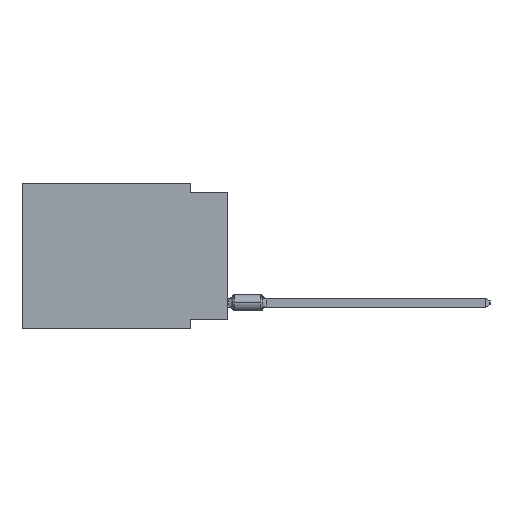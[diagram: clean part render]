
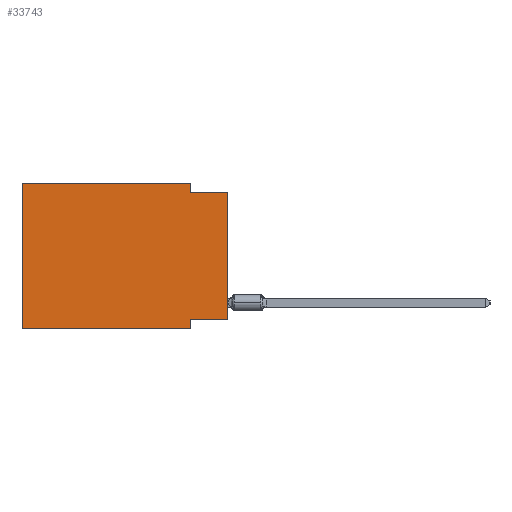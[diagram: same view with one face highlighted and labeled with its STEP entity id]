
A CAD part, left-side view. The second image highlights one B-rep face of the part: STEP entity #33743.
In plain terms, the highlighted planar face has unit normal (-1, 0, 0).
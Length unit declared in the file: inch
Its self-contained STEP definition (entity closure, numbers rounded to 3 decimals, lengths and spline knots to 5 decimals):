
#637 = CARTESIAN_POINT ( 'NONE',  ( 0., 0.55, 0. ) ) ;
#720 = DIRECTION ( 'NONE',  ( 0., 0., 1. ) ) ;
#764 = CARTESIAN_POINT ( 'NONE',  ( 0., 0.55, 0. ) ) ;
#1019 = CARTESIAN_POINT ( 'NONE',  ( 0., 0., -0.365 ) ) ;
#1382 = ORIENTED_EDGE ( 'NONE', *, *, #21105, .F. ) ;
#1525 = DIRECTION ( 'NONE',  ( 0., 0., -1. ) ) ;
#1823 = VERTEX_POINT ( 'NONE', #637 ) ;
#2099 = CARTESIAN_POINT ( 'NONE',  ( 0., 0.55, -0.39 ) ) ;
#2282 = CARTESIAN_POINT ( 'NONE',  ( 0., 0.55, 0. ) ) ;
#2800 = LINE ( 'NONE', #2282, #27940 ) ;
#3348 = LINE ( 'NONE', #8285, #8511 ) ;
#3445 = VECTOR ( 'NONE', #25038, 39.37008 ) ;
#4300 = ORIENTED_EDGE ( 'NONE', *, *, #12586, .T. ) ;
#5215 = VECTOR ( 'NONE', #23584, 39.37008 ) ;
#5415 = VERTEX_POINT ( 'NONE', #30188 ) ;
#5670 = VECTOR ( 'NONE', #11538, 39.37008 ) ;
#6249 = VECTOR ( 'NONE', #32378, 39.37008 ) ;
#6464 = EDGE_CURVE ( 'NONE', #22963, #1823, #2800, .T. ) ;
#7119 = VECTOR ( 'NONE', #720, 39.37008 ) ;
#8180 = ORIENTED_EDGE ( 'NONE', *, *, #17267, .F. ) ;
#8285 = CARTESIAN_POINT ( 'NONE',  ( 0., 0.1, -0.39 ) ) ;
#8511 = VECTOR ( 'NONE', #24791, 39.37008 ) ;
#9815 = CARTESIAN_POINT ( 'NONE',  ( 0., 0.1, 0. ) ) ;
#9948 = VERTEX_POINT ( 'NONE', #30672 ) ;
#10771 = VECTOR ( 'NONE', #1525, 39.37008 ) ;
#10955 = LINE ( 'NONE', #764, #6249 ) ;
#11538 = DIRECTION ( 'NONE',  ( 0., -1., 0. ) ) ;
#12586 = EDGE_CURVE ( 'NONE', #22963, #5415, #14336, .T. ) ;
#12925 = LINE ( 'NONE', #23476, #10771 ) ;
#13226 = LINE ( 'NONE', #26566, #5215 ) ;
#14336 = LINE ( 'NONE', #27322, #3445 ) ;
#15094 = ORIENTED_EDGE ( 'NONE', *, *, #21496, .F. ) ;
#15326 = EDGE_CURVE ( 'NONE', #25270, #18817, #27583, .T. ) ;
#15428 = PLANE ( 'NONE',  #31967 ) ;
#15624 = CARTESIAN_POINT ( 'NONE',  ( 0., 0.1, -0.365 ) ) ;
#15827 = EDGE_CURVE ( 'NONE', #24851, #9948, #12925, .T. ) ;
#15851 = EDGE_LOOP ( 'NONE', ( #25285, #20115, #17676, #1382, #32858, #4300, #15094, #8180 ) ) ;
#16592 = EDGE_CURVE ( 'NONE', #9948, #18817, #21894, .T. ) ;
#17267 = EDGE_CURVE ( 'NONE', #25270, #21760, #13226, .T. ) ;
#17676 = ORIENTED_EDGE ( 'NONE', *, *, #15827, .F. ) ;
#18791 = DIRECTION ( 'NONE',  ( 0., 0., 1. ) ) ;
#18817 = VERTEX_POINT ( 'NONE', #23208 ) ;
#20115 = ORIENTED_EDGE ( 'NONE', *, *, #16592, .F. ) ;
#21105 = EDGE_CURVE ( 'NONE', #1823, #24851, #10955, .T. ) ;
#21496 = EDGE_CURVE ( 'NONE', #21760, #5415, #3348, .T. ) ;
#21549 = CARTESIAN_POINT ( 'NONE',  ( 0., 0., -0.025 ) ) ;
#21760 = VERTEX_POINT ( 'NONE', #15624 ) ;
#21894 = LINE ( 'NONE', #21549, #5670 ) ;
#22963 = VERTEX_POINT ( 'NONE', #2099 ) ;
#23208 = CARTESIAN_POINT ( 'NONE',  ( 0., 0., -0.025 ) ) ;
#23476 = CARTESIAN_POINT ( 'NONE',  ( 0., 0.1, 0. ) ) ;
#23507 = DIRECTION ( 'NONE',  ( 1., 0., 0. ) ) ;
#23584 = DIRECTION ( 'NONE',  ( 0., 1., 0. ) ) ;
#24781 = CARTESIAN_POINT ( 'NONE',  ( 0., 0., 0. ) ) ;
#24791 = DIRECTION ( 'NONE',  ( 0., 0., -1. ) ) ;
#24851 = VERTEX_POINT ( 'NONE', #9815 ) ;
#25038 = DIRECTION ( 'NONE',  ( 0., -1., 0. ) ) ;
#25270 = VERTEX_POINT ( 'NONE', #1019 ) ;
#25285 = ORIENTED_EDGE ( 'NONE', *, *, #15326, .T. ) ;
#26566 = CARTESIAN_POINT ( 'NONE',  ( 0., 0., -0.365 ) ) ;
#27322 = CARTESIAN_POINT ( 'NONE',  ( 0., 0.55, -0.39 ) ) ;
#27583 = LINE ( 'NONE', #24781, #7119 ) ;
#27940 = VECTOR ( 'NONE', #18791, 39.37008 ) ;
#28596 = DIRECTION ( 'NONE',  ( 0., 0., -1. ) ) ;
#30188 = CARTESIAN_POINT ( 'NONE',  ( 0., 0.1, -0.39 ) ) ;
#30672 = CARTESIAN_POINT ( 'NONE',  ( 0., 0.1, -0.025 ) ) ;
#31391 = CARTESIAN_POINT ( 'NONE',  ( 0., 0.55, 0. ) ) ;
#31967 = AXIS2_PLACEMENT_3D ( 'NONE', #31391, #23507, #28596 ) ;
#32378 = DIRECTION ( 'NONE',  ( 0., -1., 0. ) ) ;
#32858 = ORIENTED_EDGE ( 'NONE', *, *, #6464, .F. ) ;
#33743 = ADVANCED_FACE ( 'NONE', ( #33853 ), #15428, .F. ) ;
#33853 = FACE_OUTER_BOUND ( 'NONE', #15851, .T. ) ;
